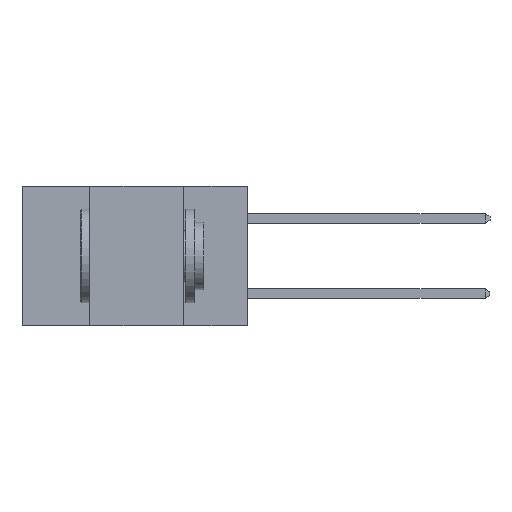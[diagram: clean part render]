
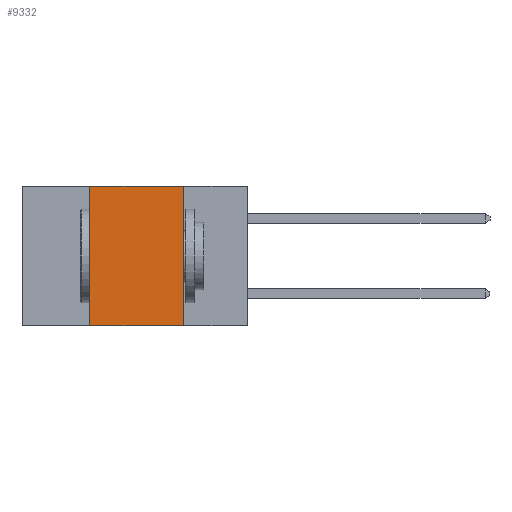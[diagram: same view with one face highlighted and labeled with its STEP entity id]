
A CAD part, left-side view. The second image highlights one B-rep face of the part: STEP entity #9332.
In plain terms, the highlighted planar face has unit normal (-1, 0, 0).
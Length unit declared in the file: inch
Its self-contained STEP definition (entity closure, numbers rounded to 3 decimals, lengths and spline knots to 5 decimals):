
#446 = CARTESIAN_POINT ( 'NONE',  ( 0., 0.6, 0. ) ) ;
#909 = CARTESIAN_POINT ( 'NONE',  ( 0., 0.42, 0. ) ) ;
#931 = ORIENTED_EDGE ( 'NONE', *, *, #8024, .F. ) ;
#1217 = CARTESIAN_POINT ( 'NONE',  ( 0., 0.17, 0. ) ) ;
#1218 = ORIENTED_EDGE ( 'NONE', *, *, #9627, .T. ) ;
#1432 = VERTEX_POINT ( 'NONE', #1217 ) ;
#1927 = CARTESIAN_POINT ( 'NONE',  ( 0., 0.17, 0. ) ) ;
#1988 = LINE ( 'NONE', #446, #6141 ) ;
#2095 = FACE_OUTER_BOUND ( 'NONE', #6569, .T. ) ;
#2438 = DIRECTION ( 'NONE',  ( 1., 0., 0. ) ) ;
#2592 = AXIS2_PLACEMENT_3D ( 'NONE', #4071, #2438, #8222 ) ;
#2716 = CARTESIAN_POINT ( 'NONE',  ( 0., 0.17, -0.37 ) ) ;
#2795 = DIRECTION ( 'NONE',  ( 0., 0., -1. ) ) ;
#3270 = DIRECTION ( 'NONE',  ( 0., 0., 1. ) ) ;
#3413 = VECTOR ( 'NONE', #6924, 39.37008 ) ;
#3786 = VERTEX_POINT ( 'NONE', #2716 ) ;
#4071 = CARTESIAN_POINT ( 'NONE',  ( 0., 0.6, 0. ) ) ;
#4669 = DIRECTION ( 'NONE',  ( 0., -1., 0. ) ) ;
#5154 = ORIENTED_EDGE ( 'NONE', *, *, #9643, .F. ) ;
#5593 = LINE ( 'NONE', #1927, #7555 ) ;
#6056 = CARTESIAN_POINT ( 'NONE',  ( 0., 0.6, -0.37 ) ) ;
#6141 = VECTOR ( 'NONE', #4669, 39.37008 ) ;
#6365 = VERTEX_POINT ( 'NONE', #909 ) ;
#6512 = LINE ( 'NONE', #9084, #10351 ) ;
#6569 = EDGE_LOOP ( 'NONE', ( #5154, #931, #9801, #1218 ) ) ;
#6924 = DIRECTION ( 'NONE',  ( 0., -1., 0. ) ) ;
#7555 = VECTOR ( 'NONE', #2795, 39.37008 ) ;
#7830 = LINE ( 'NONE', #6056, #3413 ) ;
#8024 = EDGE_CURVE ( 'NONE', #6365, #1432, #1988, .T. ) ;
#8147 = VERTEX_POINT ( 'NONE', #9744 ) ;
#8182 = PLANE ( 'NONE',  #2592 ) ;
#8222 = DIRECTION ( 'NONE',  ( 0., 0., -1. ) ) ;
#9084 = CARTESIAN_POINT ( 'NONE',  ( 0., 0.42, 0. ) ) ;
#9332 = ADVANCED_FACE ( 'NONE', ( #2095 ), #8182, .F. ) ;
#9335 = EDGE_CURVE ( 'NONE', #8147, #6365, #6512, .T. ) ;
#9627 = EDGE_CURVE ( 'NONE', #8147, #3786, #7830, .T. ) ;
#9643 = EDGE_CURVE ( 'NONE', #1432, #3786, #5593, .T. ) ;
#9744 = CARTESIAN_POINT ( 'NONE',  ( 0., 0.42, -0.37 ) ) ;
#9801 = ORIENTED_EDGE ( 'NONE', *, *, #9335, .F. ) ;
#10351 = VECTOR ( 'NONE', #3270, 39.37008 ) ;
